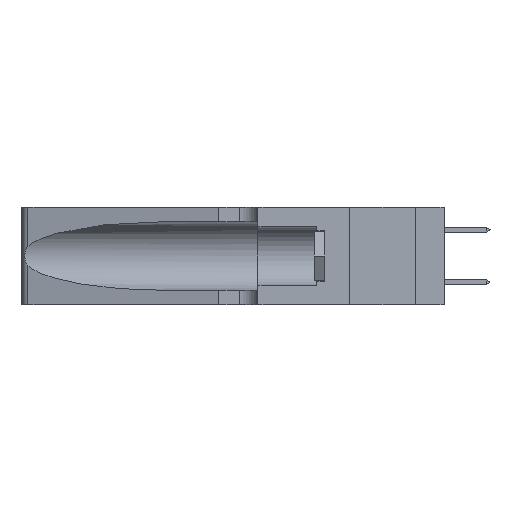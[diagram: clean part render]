
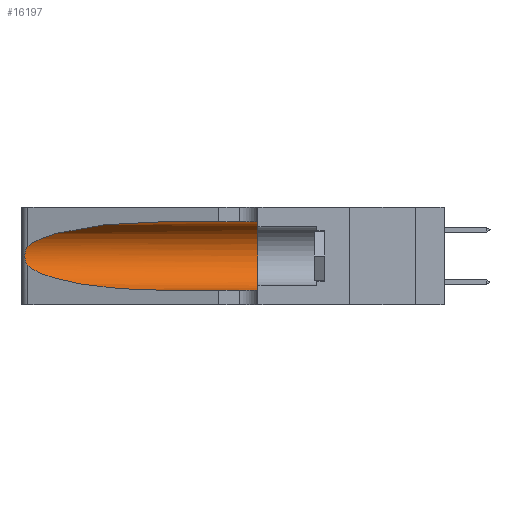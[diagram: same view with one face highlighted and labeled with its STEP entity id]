
A CAD part, left-side view. The second image highlights one B-rep face of the part: STEP entity #16197.
In plain terms, the highlighted cylindrical face has radius 3.308 mm (diameter 6.617 mm), a partial arc.
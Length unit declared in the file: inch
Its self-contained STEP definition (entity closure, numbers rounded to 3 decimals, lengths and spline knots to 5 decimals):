
#20 = CARTESIAN_POINT ( 'NONE',  ( 0.25789, 1.23486, 0.15765 ) ) ;
#1305 = ORIENTED_EDGE ( 'NONE', *, *, #13160, .T. ) ;
#2298 = CIRCLE ( 'NONE', #9800, 0.13025 ) ;
#2912 = CARTESIAN_POINT ( 'NONE',  ( 0.25639, 1.23184, 0.21858 ) ) ;
#3037 = CARTESIAN_POINT ( 'NONE',  ( 0.25787, 1.23484, 0.2124 ) ) ;
#3043 =( BOUNDED_CURVE ( )  B_SPLINE_CURVE ( 3, ( #34248, #17955, #34864, #34984 ),
 .UNSPECIFIED., .F., .T. ) 
 B_SPLINE_CURVE_WITH_KNOTS ( ( 4, 4 ),
 ( 1.5708, 2.84003 ),
 .UNSPECIFIED. ) 
 CURVE ( )  GEOMETRIC_REPRESENTATION_ITEM ( )  RATIONAL_B_SPLINE_CURVE ( ( 1., 0.87, 0.87, 1. ) ) 
 REPRESENTATION_ITEM ( '' )  );
#3206 = DIRECTION ( 'NONE',  ( 0., 1., 0. ) ) ;
#3939 = VERTEX_POINT ( 'NONE', #16581 ) ;
#4119 = CARTESIAN_POINT ( 'NONE',  ( 0.1305, 0.72297, 0.05475 ) ) ;
#4161 = B_SPLINE_CURVE_WITH_KNOTS ( 'NONE', 3,
 ( #17265, #22979, #2912, #3037, #29257, #5671, #29012, #14350, #17515, #31911, #20, #36790, #8693, #14718 ),
 .UNSPECIFIED., .F., .F.,
 ( 4, 2, 2, 2, 2, 2, 4 ),
 ( 0., 0.00027, 0.00053, 0.00107, 0.0016, 0.00187, 0.00214 ),
 .UNSPECIFIED. ) ;
#5098 = ORIENTED_EDGE ( 'NONE', *, *, #28160, .T. ) ;
#5671 = CARTESIAN_POINT ( 'NONE',  ( 0.26018, 1.23835, 0.19895 ) ) ;
#5818 = CARTESIAN_POINT ( 'NONE',  ( 0.1305, 0.72297, 0.31525 ) ) ;
#5996 =( BOUNDED_CURVE ( )  B_SPLINE_CURVE ( 3, ( #19000, #27854, #36145, #21924 ),
 .UNSPECIFIED., .F., .F. ) 
 B_SPLINE_CURVE_WITH_KNOTS ( ( 4, 4 ),
 ( 3.44316, 4.71239 ),
 .UNSPECIFIED. ) 
 CURVE ( )  GEOMETRIC_REPRESENTATION_ITEM ( )  RATIONAL_B_SPLINE_CURVE ( ( 1., 0.87, 0.87, 1. ) ) 
 REPRESENTATION_ITEM ( '' )  );
#6428 = DIRECTION ( 'NONE',  ( 0., -1., 0. ) ) ;
#7623 = CARTESIAN_POINT ( 'NONE',  ( 0.1305, 1.61858, 0.05475 ) ) ;
#7738 = ORIENTED_EDGE ( 'NONE', *, *, #14804, .T. ) ;
#8580 = CARTESIAN_POINT ( 'NONE',  ( 0.1305, 1.61858, 0.185 ) ) ;
#8693 = CARTESIAN_POINT ( 'NONE',  ( 0.25555, 1.22993, 0.14849 ) ) ;
#9800 = AXIS2_PLACEMENT_3D ( 'NONE', #11635, #3206, #23153 ) ;
#11635 = CARTESIAN_POINT ( 'NONE',  ( 0.1305, 0.35, 0.185 ) ) ;
#12204 = DIRECTION ( 'NONE',  ( 0., 0., -1. ) ) ;
#12946 = DIRECTION ( 'NONE',  ( 0., -1., 0. ) ) ;
#13160 = EDGE_CURVE ( 'NONE', #26973, #25390, #3043, .T. ) ;
#13339 = CARTESIAN_POINT ( 'NONE',  ( 0.1305, 1.61858, 0.31525 ) ) ;
#13541 = DIRECTION ( 'NONE',  ( 0., -1., 0. ) ) ;
#13657 = VECTOR ( 'NONE', #12946, 39.37008 ) ;
#14350 = CARTESIAN_POINT ( 'NONE',  ( 0.26075, 1.23896, 0.178 ) ) ;
#14406 = AXIS2_PLACEMENT_3D ( 'NONE', #8580, #6428, #12204 ) ;
#14555 = LINE ( 'NONE', #13339, #13657 ) ;
#14718 = CARTESIAN_POINT ( 'NONE',  ( 0.25487, 1.22718, 0.14631 ) ) ;
#14804 = EDGE_CURVE ( 'NONE', #30504, #29594, #32786, .T. ) ;
#16197 = ADVANCED_FACE ( 'NONE', ( #20537 ), #30002, .F. ) ;
#16581 = CARTESIAN_POINT ( 'NONE',  ( 0.25487, 1.22718, 0.14631 ) ) ;
#17005 = EDGE_CURVE ( 'NONE', #26973, #24520, #14555, .T. ) ;
#17265 = CARTESIAN_POINT ( 'NONE',  ( 0.25487, 1.22718, 0.22369 ) ) ;
#17515 = CARTESIAN_POINT ( 'NONE',  ( 0.26017, 1.23833, 0.17102 ) ) ;
#17741 = EDGE_LOOP ( 'NONE', ( #1305, #5098, #24084, #7738, #21741, #29834 ) ) ;
#17955 = CARTESIAN_POINT ( 'NONE',  ( 0.18966, 0.96281, 0.31525 ) ) ;
#19000 = CARTESIAN_POINT ( 'NONE',  ( 0.25487, 1.22718, 0.14631 ) ) ;
#20537 = FACE_OUTER_BOUND ( 'NONE', #17741, .T. ) ;
#21741 = ORIENTED_EDGE ( 'NONE', *, *, #23326, .F. ) ;
#21924 = CARTESIAN_POINT ( 'NONE',  ( 0.1305, 0.72297, 0.05475 ) ) ;
#22979 = CARTESIAN_POINT ( 'NONE',  ( 0.25555, 1.22994, 0.2215 ) ) ;
#23153 = DIRECTION ( 'NONE',  ( 0., 0., 1. ) ) ;
#23326 = EDGE_CURVE ( 'NONE', #24520, #29594, #2298, .T. ) ;
#24084 = ORIENTED_EDGE ( 'NONE', *, *, #32437, .T. ) ;
#24520 = VERTEX_POINT ( 'NONE', #25090 ) ;
#25090 = CARTESIAN_POINT ( 'NONE',  ( 0.1305, 0.35, 0.31525 ) ) ;
#25390 = VERTEX_POINT ( 'NONE', #36057 ) ;
#26515 = CARTESIAN_POINT ( 'NONE',  ( 0.1305, 0.35, 0.05475 ) ) ;
#26948 = VECTOR ( 'NONE', #13541, 39.37008 ) ;
#26973 = VERTEX_POINT ( 'NONE', #5818 ) ;
#27854 = CARTESIAN_POINT ( 'NONE',  ( 0.2373, 1.15595, 0.08982 ) ) ;
#28160 = EDGE_CURVE ( 'NONE', #25390, #3939, #4161, .T. ) ;
#29012 = CARTESIAN_POINT ( 'NONE',  ( 0.26075, 1.23896, 0.19203 ) ) ;
#29257 = CARTESIAN_POINT ( 'NONE',  ( 0.25854, 1.2359, 0.20912 ) ) ;
#29594 = VERTEX_POINT ( 'NONE', #26515 ) ;
#29834 = ORIENTED_EDGE ( 'NONE', *, *, #17005, .F. ) ;
#30002 = CYLINDRICAL_SURFACE ( 'NONE', #14406, 0.13025 ) ;
#30504 = VERTEX_POINT ( 'NONE', #4119 ) ;
#31911 = CARTESIAN_POINT ( 'NONE',  ( 0.25856, 1.23593, 0.16098 ) ) ;
#32437 = EDGE_CURVE ( 'NONE', #3939, #30504, #5996, .T. ) ;
#32786 = LINE ( 'NONE', #7623, #26948 ) ;
#34248 = CARTESIAN_POINT ( 'NONE',  ( 0.1305, 0.72297, 0.31525 ) ) ;
#34864 = CARTESIAN_POINT ( 'NONE',  ( 0.2373, 1.15595, 0.28018 ) ) ;
#34984 = CARTESIAN_POINT ( 'NONE',  ( 0.25487, 1.22718, 0.22369 ) ) ;
#36057 = CARTESIAN_POINT ( 'NONE',  ( 0.25487, 1.22718, 0.22369 ) ) ;
#36145 = CARTESIAN_POINT ( 'NONE',  ( 0.18966, 0.96281, 0.05475 ) ) ;
#36790 = CARTESIAN_POINT ( 'NONE',  ( 0.25639, 1.23186, 0.15144 ) ) ;
